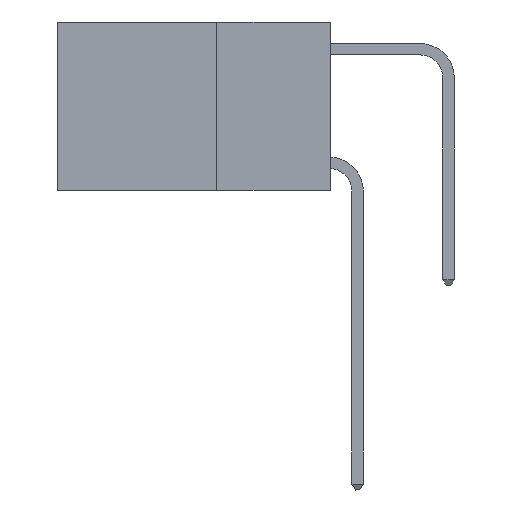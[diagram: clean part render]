
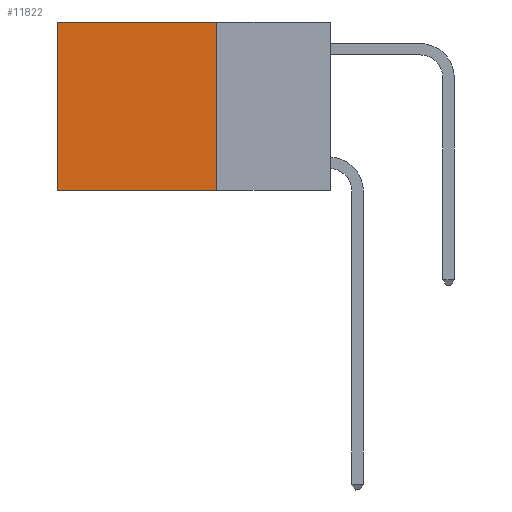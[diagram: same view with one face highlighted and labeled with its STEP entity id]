
A CAD part, left-side view. The second image highlights one B-rep face of the part: STEP entity #11822.
In plain terms, the highlighted planar face has unit normal (-1, 0, 0).
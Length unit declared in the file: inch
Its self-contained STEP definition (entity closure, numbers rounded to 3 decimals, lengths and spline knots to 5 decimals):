
#333 = LINE ( 'NONE', #13673, #3589 ) ;
#1415 = LINE ( 'NONE', #8023, #13209 ) ;
#1457 = CARTESIAN_POINT ( 'NONE',  ( 0.2625, 0.6, 0. ) ) ;
#2404 = CARTESIAN_POINT ( 'NONE',  ( 0.2625, 0.25, 0. ) ) ;
#2817 = CARTESIAN_POINT ( 'NONE',  ( 0.2625, 0.25, -0.37 ) ) ;
#2864 = DIRECTION ( 'NONE',  ( 0., 0., -1. ) ) ;
#3027 = VERTEX_POINT ( 'NONE', #19807 ) ;
#3326 = VERTEX_POINT ( 'NONE', #17824 ) ;
#3468 = ORIENTED_EDGE ( 'NONE', *, *, #15590, .T. ) ;
#3589 = VECTOR ( 'NONE', #3780, 39.37008 ) ;
#3725 = EDGE_LOOP ( 'NONE', ( #3468, #15720, #12890, #13913 ) ) ;
#3780 = DIRECTION ( 'NONE',  ( 0., 1., 0. ) ) ;
#4309 = EDGE_CURVE ( 'NONE', #3326, #11280, #333, .T. ) ;
#5453 = DIRECTION ( 'NONE',  ( 0., 0., -1. ) ) ;
#5754 = VECTOR ( 'NONE', #2864, 39.37008 ) ;
#5781 = VECTOR ( 'NONE', #6242, 39.37008 ) ;
#6242 = DIRECTION ( 'NONE',  ( 0., 1., 0. ) ) ;
#7308 = LINE ( 'NONE', #1457, #5754 ) ;
#8023 = CARTESIAN_POINT ( 'NONE',  ( 0.2625, 0.25, 0. ) ) ;
#8591 = EDGE_CURVE ( 'NONE', #3326, #13922, #1415, .T. ) ;
#9020 = PLANE ( 'NONE',  #19475 ) ;
#9512 = CARTESIAN_POINT ( 'NONE',  ( 0.2625, 0.6, 0. ) ) ;
#11280 = VERTEX_POINT ( 'NONE', #9512 ) ;
#11822 = ADVANCED_FACE ( 'NONE', ( #20389 ), #9020, .F. ) ;
#12810 = DIRECTION ( 'NONE',  ( 1., 0., 0. ) ) ;
#12890 = ORIENTED_EDGE ( 'NONE', *, *, #8591, .F. ) ;
#13209 = VECTOR ( 'NONE', #21212, 39.37008 ) ;
#13673 = CARTESIAN_POINT ( 'NONE',  ( 0.2625, 0.25, 0. ) ) ;
#13913 = ORIENTED_EDGE ( 'NONE', *, *, #4309, .T. ) ;
#13922 = VERTEX_POINT ( 'NONE', #2817 ) ;
#15590 = EDGE_CURVE ( 'NONE', #11280, #3027, #7308, .T. ) ;
#15720 = ORIENTED_EDGE ( 'NONE', *, *, #17107, .F. ) ;
#17107 = EDGE_CURVE ( 'NONE', #13922, #3027, #17600, .T. ) ;
#17600 = LINE ( 'NONE', #19449, #5781 ) ;
#17824 = CARTESIAN_POINT ( 'NONE',  ( 0.2625, 0.25, 0. ) ) ;
#19449 = CARTESIAN_POINT ( 'NONE',  ( 0.2625, 0.25, -0.37 ) ) ;
#19475 = AXIS2_PLACEMENT_3D ( 'NONE', #2404, #12810, #5453 ) ;
#19807 = CARTESIAN_POINT ( 'NONE',  ( 0.2625, 0.6, -0.37 ) ) ;
#20389 = FACE_OUTER_BOUND ( 'NONE', #3725, .T. ) ;
#21212 = DIRECTION ( 'NONE',  ( 0., 0., -1. ) ) ;
